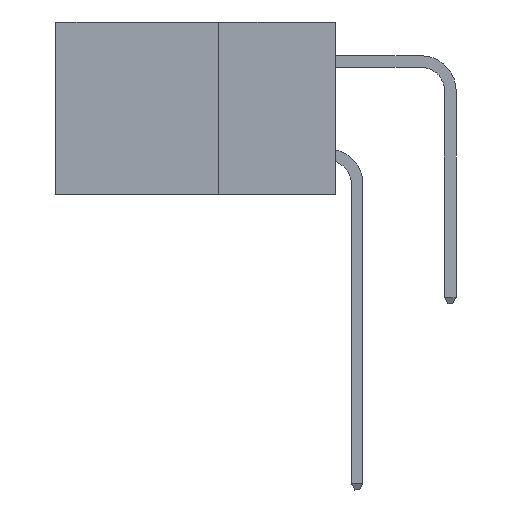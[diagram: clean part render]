
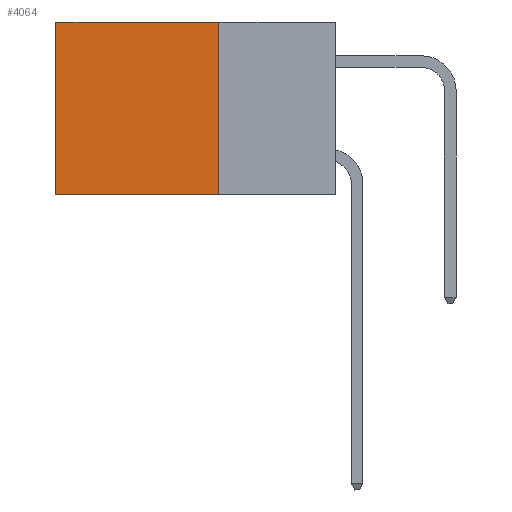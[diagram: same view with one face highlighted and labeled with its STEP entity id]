
A CAD part, left-side view. The second image highlights one B-rep face of the part: STEP entity #4064.
In plain terms, the highlighted planar face has unit normal (-1, 0, 0).
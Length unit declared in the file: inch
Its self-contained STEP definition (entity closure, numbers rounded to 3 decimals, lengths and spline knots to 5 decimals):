
#93 = EDGE_CURVE ( 'NONE', #3461, #13407, #11893, .T. ) ;
#1063 = LINE ( 'NONE', #12747, #5308 ) ;
#1658 = DIRECTION ( 'NONE',  ( 1., 0., 0. ) ) ;
#1682 = DIRECTION ( 'NONE',  ( 0., 1., 0. ) ) ;
#3461 = VERTEX_POINT ( 'NONE', #14939 ) ;
#3540 = VECTOR ( 'NONE', #18930, 39.37008 ) ;
#3669 = VERTEX_POINT ( 'NONE', #11648 ) ;
#4064 = ADVANCED_FACE ( 'NONE', ( #14207 ), #4290, .F. ) ;
#4108 = ORIENTED_EDGE ( 'NONE', *, *, #10231, .F. ) ;
#4290 = PLANE ( 'NONE',  #8492 ) ;
#4395 = EDGE_CURVE ( 'NONE', #13407, #3669, #7797, .T. ) ;
#5238 = EDGE_CURVE ( 'NONE', #3461, #11106, #7757, .T. ) ;
#5308 = VECTOR ( 'NONE', #1682, 39.37008 ) ;
#6256 = EDGE_LOOP ( 'NONE', ( #18835, #4108, #12502, #9840 ) ) ;
#7257 = VECTOR ( 'NONE', #18367, 39.37008 ) ;
#7757 = LINE ( 'NONE', #10526, #7257 ) ;
#7797 = LINE ( 'NONE', #19682, #3540 ) ;
#8492 = AXIS2_PLACEMENT_3D ( 'NONE', #9872, #1658, #14485 ) ;
#9840 = ORIENTED_EDGE ( 'NONE', *, *, #93, .T. ) ;
#9872 = CARTESIAN_POINT ( 'NONE',  ( 0.2875, 0.25, 0. ) ) ;
#10231 = EDGE_CURVE ( 'NONE', #11106, #3669, #1063, .T. ) ;
#10526 = CARTESIAN_POINT ( 'NONE',  ( 0.2875, 0.25, 0. ) ) ;
#11106 = VERTEX_POINT ( 'NONE', #11637 ) ;
#11637 = CARTESIAN_POINT ( 'NONE',  ( 0.2875, 0.25, -0.37 ) ) ;
#11648 = CARTESIAN_POINT ( 'NONE',  ( 0.2875, 0.6, -0.37 ) ) ;
#11893 = LINE ( 'NONE', #14889, #19680 ) ;
#12502 = ORIENTED_EDGE ( 'NONE', *, *, #5238, .F. ) ;
#12747 = CARTESIAN_POINT ( 'NONE',  ( 0.2875, 0.25, -0.37 ) ) ;
#13407 = VERTEX_POINT ( 'NONE', #15840 ) ;
#14207 = FACE_OUTER_BOUND ( 'NONE', #6256, .T. ) ;
#14485 = DIRECTION ( 'NONE',  ( 0., 0., -1. ) ) ;
#14682 = DIRECTION ( 'NONE',  ( 0., 1., 0. ) ) ;
#14889 = CARTESIAN_POINT ( 'NONE',  ( 0.2875, 0.25, 0. ) ) ;
#14939 = CARTESIAN_POINT ( 'NONE',  ( 0.2875, 0.25, 0. ) ) ;
#15840 = CARTESIAN_POINT ( 'NONE',  ( 0.2875, 0.6, 0. ) ) ;
#18367 = DIRECTION ( 'NONE',  ( 0., 0., -1. ) ) ;
#18835 = ORIENTED_EDGE ( 'NONE', *, *, #4395, .T. ) ;
#18930 = DIRECTION ( 'NONE',  ( 0., 0., -1. ) ) ;
#19680 = VECTOR ( 'NONE', #14682, 39.37008 ) ;
#19682 = CARTESIAN_POINT ( 'NONE',  ( 0.2875, 0.6, 0. ) ) ;
